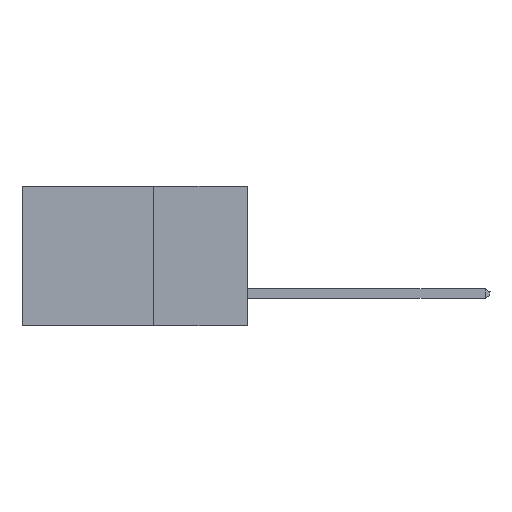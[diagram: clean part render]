
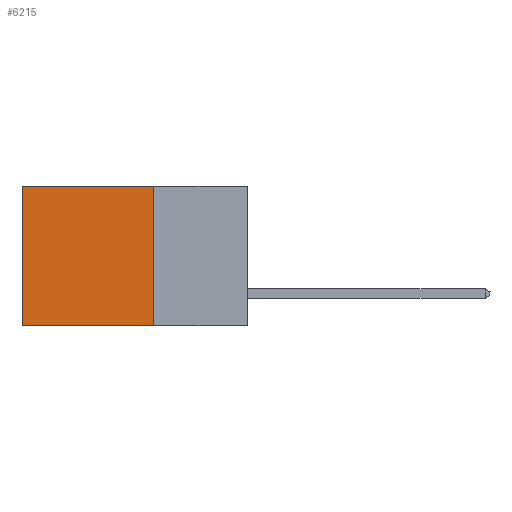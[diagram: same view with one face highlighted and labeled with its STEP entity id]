
A CAD part, left-side view. The second image highlights one B-rep face of the part: STEP entity #6215.
In plain terms, the highlighted planar face has unit normal (-1, 0, 0).
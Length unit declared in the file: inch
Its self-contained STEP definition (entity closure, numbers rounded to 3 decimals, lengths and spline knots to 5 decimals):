
#1330 = LINE ( 'NONE', #1454, #17229 ) ;
#1454 = CARTESIAN_POINT ( 'NONE',  ( 0.2615, 0.25, -0.37 ) ) ;
#1746 = VERTEX_POINT ( 'NONE', #17213 ) ;
#1847 = VERTEX_POINT ( 'NONE', #25146 ) ;
#2394 = VECTOR ( 'NONE', #9670, 39.37008 ) ;
#3914 = LINE ( 'NONE', #23301, #2394 ) ;
#4599 = ORIENTED_EDGE ( 'NONE', *, *, #10544, .F. ) ;
#4765 = CARTESIAN_POINT ( 'NONE',  ( 0.2615, 0.6, -0.37 ) ) ;
#5147 = LINE ( 'NONE', #4765, #23369 ) ;
#5408 = LINE ( 'NONE', #20704, #17776 ) ;
#5437 = DIRECTION ( 'NONE',  ( 0., 1., 0. ) ) ;
#6215 = ADVANCED_FACE ( 'NONE', ( #12838 ), #18604, .F. ) ;
#6397 = EDGE_CURVE ( 'NONE', #10233, #1847, #5408, .T. ) ;
#7068 = DIRECTION ( 'NONE',  ( 0., 0., -1. ) ) ;
#8440 = ORIENTED_EDGE ( 'NONE', *, *, #24502, .T. ) ;
#8925 = DIRECTION ( 'NONE',  ( 0., 0., -1. ) ) ;
#9670 = DIRECTION ( 'NONE',  ( 0., 0., -1. ) ) ;
#10046 = AXIS2_PLACEMENT_3D ( 'NONE', #15133, #11062, #8925 ) ;
#10233 = VERTEX_POINT ( 'NONE', #21242 ) ;
#10544 = EDGE_CURVE ( 'NONE', #10233, #1746, #3914, .T. ) ;
#11062 = DIRECTION ( 'NONE',  ( 1., 0., 0. ) ) ;
#12838 = FACE_OUTER_BOUND ( 'NONE', #13438, .T. ) ;
#13438 = EDGE_LOOP ( 'NONE', ( #8440, #16370, #4599, #19537 ) ) ;
#15133 = CARTESIAN_POINT ( 'NONE',  ( 0.2615, 0.25, -0.37 ) ) ;
#16370 = ORIENTED_EDGE ( 'NONE', *, *, #24731, .F. ) ;
#17213 = CARTESIAN_POINT ( 'NONE',  ( 0.2615, 0.25, -0.37 ) ) ;
#17229 = VECTOR ( 'NONE', #5437, 39.37008 ) ;
#17776 = VECTOR ( 'NONE', #22498, 39.37008 ) ;
#18604 = PLANE ( 'NONE',  #10046 ) ;
#18663 = CARTESIAN_POINT ( 'NONE',  ( 0.2615, 0.6, -0.37 ) ) ;
#19537 = ORIENTED_EDGE ( 'NONE', *, *, #6397, .T. ) ;
#20704 = CARTESIAN_POINT ( 'NONE',  ( 0.2615, 0.25, 0. ) ) ;
#21242 = CARTESIAN_POINT ( 'NONE',  ( 0.2615, 0.25, 0. ) ) ;
#22498 = DIRECTION ( 'NONE',  ( 0., 1., 0. ) ) ;
#23301 = CARTESIAN_POINT ( 'NONE',  ( 0.2615, 0.25, -0.37 ) ) ;
#23369 = VECTOR ( 'NONE', #7068, 39.37008 ) ;
#24502 = EDGE_CURVE ( 'NONE', #1847, #24517, #5147, .T. ) ;
#24517 = VERTEX_POINT ( 'NONE', #18663 ) ;
#24731 = EDGE_CURVE ( 'NONE', #1746, #24517, #1330, .T. ) ;
#25146 = CARTESIAN_POINT ( 'NONE',  ( 0.2615, 0.6, 0. ) ) ;
